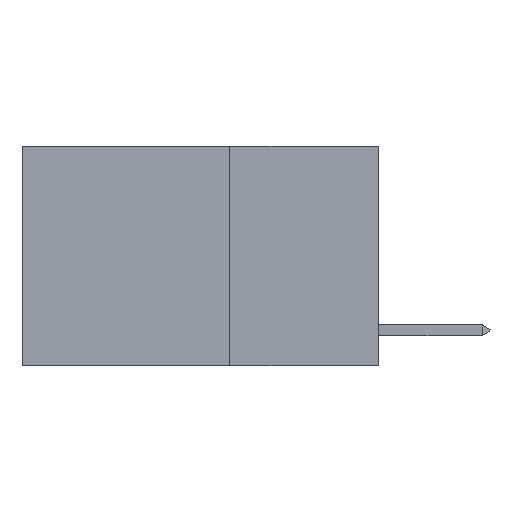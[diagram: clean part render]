
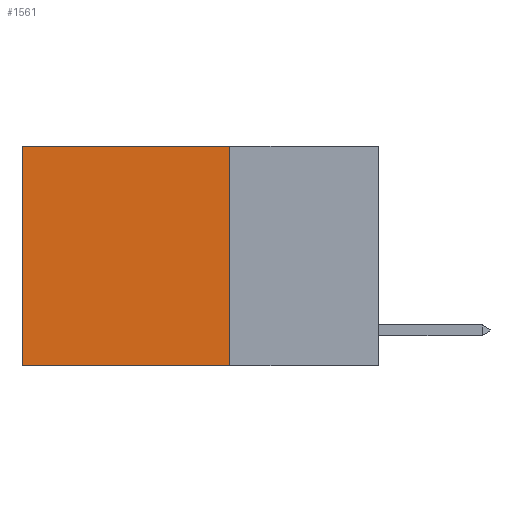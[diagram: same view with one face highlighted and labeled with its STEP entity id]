
A CAD part, left-side view. The second image highlights one B-rep face of the part: STEP entity #1561.
In plain terms, the highlighted planar face has unit normal (-1, 0, 0).
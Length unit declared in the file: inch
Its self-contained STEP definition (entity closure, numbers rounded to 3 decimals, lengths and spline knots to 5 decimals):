
#380 = ORIENTED_EDGE ( 'NONE', *, *, #10611, .T. ) ;
#407 = ORIENTED_EDGE ( 'NONE', *, *, #9455, .T. ) ;
#599 = EDGE_CURVE ( 'NONE', #12261, #9765, #3262, .T. ) ;
#1312 = DIRECTION ( 'NONE',  ( 0., 1., 0. ) ) ;
#1397 = CARTESIAN_POINT ( 'NONE',  ( 0.2625, 0.6, 0. ) ) ;
#1561 = ADVANCED_FACE ( 'NONE', ( #13477 ), #7748, .F. ) ;
#2203 = LINE ( 'NONE', #3027, #2566 ) ;
#2383 = LINE ( 'NONE', #10871, #4442 ) ;
#2419 = VECTOR ( 'NONE', #11679, 39.37008 ) ;
#2566 = VECTOR ( 'NONE', #4225, 39.37008 ) ;
#3027 = CARTESIAN_POINT ( 'NONE',  ( 0.2625, 0.25, 0. ) ) ;
#3080 = CARTESIAN_POINT ( 'NONE',  ( 0.2625, 0.6, -0.37 ) ) ;
#3262 = LINE ( 'NONE', #8869, #6071 ) ;
#4225 = DIRECTION ( 'NONE',  ( 0., 0., -1. ) ) ;
#4442 = VECTOR ( 'NONE', #4928, 39.37008 ) ;
#4468 = ORIENTED_EDGE ( 'NONE', *, *, #5442, .F. ) ;
#4551 = CARTESIAN_POINT ( 'NONE',  ( 0.2625, 0.25, 0. ) ) ;
#4928 = DIRECTION ( 'NONE',  ( 0., 0., -1. ) ) ;
#5442 = EDGE_CURVE ( 'NONE', #7854, #12261, #2203, .T. ) ;
#6071 = VECTOR ( 'NONE', #1312, 39.37008 ) ;
#7448 = DIRECTION ( 'NONE',  ( 0., 0., -1. ) ) ;
#7484 = DIRECTION ( 'NONE',  ( 1., 0., 0. ) ) ;
#7509 = CARTESIAN_POINT ( 'NONE',  ( 0.2625, 0.25, 0. ) ) ;
#7748 = PLANE ( 'NONE',  #9476 ) ;
#7826 = EDGE_LOOP ( 'NONE', ( #380, #14302, #4468, #407 ) ) ;
#7854 = VERTEX_POINT ( 'NONE', #9060 ) ;
#8869 = CARTESIAN_POINT ( 'NONE',  ( 0.2625, 0.25, -0.37 ) ) ;
#9060 = CARTESIAN_POINT ( 'NONE',  ( 0.2625, 0.25, 0. ) ) ;
#9455 = EDGE_CURVE ( 'NONE', #7854, #10097, #15016, .T. ) ;
#9476 = AXIS2_PLACEMENT_3D ( 'NONE', #7509, #7484, #7448 ) ;
#9765 = VERTEX_POINT ( 'NONE', #3080 ) ;
#10097 = VERTEX_POINT ( 'NONE', #1397 ) ;
#10611 = EDGE_CURVE ( 'NONE', #10097, #9765, #2383, .T. ) ;
#10871 = CARTESIAN_POINT ( 'NONE',  ( 0.2625, 0.6, 0. ) ) ;
#11679 = DIRECTION ( 'NONE',  ( 0., 1., 0. ) ) ;
#12261 = VERTEX_POINT ( 'NONE', #12606 ) ;
#12606 = CARTESIAN_POINT ( 'NONE',  ( 0.2625, 0.25, -0.37 ) ) ;
#13477 = FACE_OUTER_BOUND ( 'NONE', #7826, .T. ) ;
#14302 = ORIENTED_EDGE ( 'NONE', *, *, #599, .F. ) ;
#15016 = LINE ( 'NONE', #4551, #2419 ) ;
